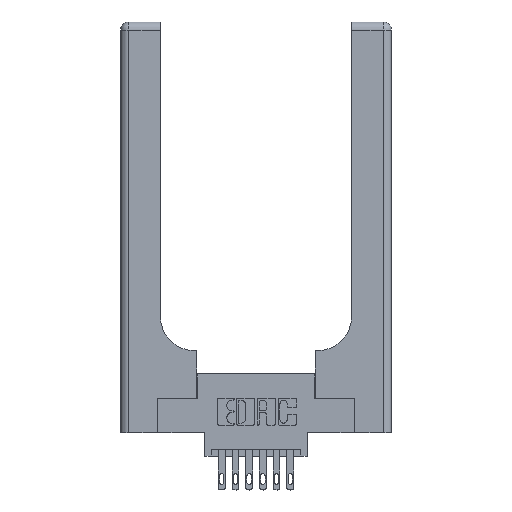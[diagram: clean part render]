
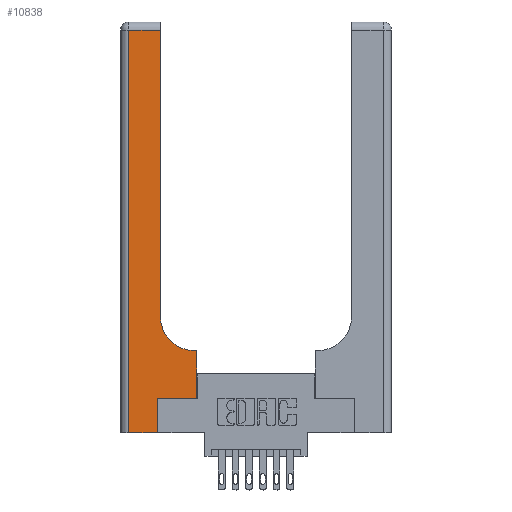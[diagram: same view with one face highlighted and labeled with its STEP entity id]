
A CAD part, top view. The second image highlights one B-rep face of the part: STEP entity #10838.
In plain terms, the highlighted planar face has unit normal (0, 0, 1).
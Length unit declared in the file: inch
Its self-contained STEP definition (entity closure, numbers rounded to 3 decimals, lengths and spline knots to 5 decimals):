
#20 = CARTESIAN_POINT ( 'NONE',  ( 0.2915, 0.6, 0.37 ) ) ;
#123 = PLANE ( 'NONE',  #11842 ) ;
#277 = CARTESIAN_POINT ( 'NONE',  ( 0.06, 0., 0.37 ) ) ;
#364 = EDGE_CURVE ( 'NONE', #12916, #10459, #4195, .T. ) ;
#506 = VECTOR ( 'NONE', #4941, 39.37008 ) ;
#641 = DIRECTION ( 'NONE',  ( 0., 1., 0. ) ) ;
#642 = EDGE_CURVE ( 'NONE', #7606, #8625, #7734, .T. ) ;
#689 = ORIENTED_EDGE ( 'NONE', *, *, #13143, .T. ) ;
#732 = VECTOR ( 'NONE', #7771, 39.37008 ) ;
#889 = DIRECTION ( 'NONE',  ( -1., 0., 0. ) ) ;
#1004 = ORIENTED_EDGE ( 'NONE', *, *, #14574, .T. ) ;
#1113 = VECTOR ( 'NONE', #1966, 39.37008 ) ;
#1472 = CARTESIAN_POINT ( 'NONE',  ( 0.5415, 0.6, 0.37 ) ) ;
#1966 = DIRECTION ( 'NONE',  ( 1., 0., 0. ) ) ;
#2055 = ORIENTED_EDGE ( 'NONE', *, *, #12424, .T. ) ;
#2529 = VECTOR ( 'NONE', #12129, 39.37008 ) ;
#2734 = VERTEX_POINT ( 'NONE', #10168 ) ;
#2869 = ORIENTED_EDGE ( 'NONE', *, *, #642, .T. ) ;
#3172 = EDGE_CURVE ( 'NONE', #13018, #13622, #7859, .T. ) ;
#3387 = CARTESIAN_POINT ( 'NONE',  ( 0.269, 0., 0.37 ) ) ;
#4195 = CIRCLE ( 'NONE', #6456, 0.25 ) ;
#4466 = VECTOR ( 'NONE', #641, 39.37008 ) ;
#4496 = LINE ( 'NONE', #20, #12321 ) ;
#4925 = CARTESIAN_POINT ( 'NONE',  ( 0.5585, 0.25, 0.37 ) ) ;
#4941 = DIRECTION ( 'NONE',  ( 1., 0., 0. ) ) ;
#5006 = LINE ( 'NONE', #11757, #506 ) ;
#5586 = LINE ( 'NONE', #11095, #732 ) ;
#5652 = DIRECTION ( 'NONE',  ( 1., 0., 0. ) ) ;
#6067 = LINE ( 'NONE', #12488, #12828 ) ;
#6456 = AXIS2_PLACEMENT_3D ( 'NONE', #11412, #7791, #5652 ) ;
#6542 = ORIENTED_EDGE ( 'NONE', *, *, #14166, .T. ) ;
#7606 = VERTEX_POINT ( 'NONE', #277 ) ;
#7608 = CARTESIAN_POINT ( 'NONE',  ( 0.06, 3., 0.37 ) ) ;
#7734 = LINE ( 'NONE', #13352, #1113 ) ;
#7771 = DIRECTION ( 'NONE',  ( 0., 1., 0. ) ) ;
#7791 = DIRECTION ( 'NONE',  ( 0., 0., -1. ) ) ;
#7859 = LINE ( 'NONE', #10879, #4466 ) ;
#8048 = DIRECTION ( 'NONE',  ( -1., 0., 0. ) ) ;
#8280 = CARTESIAN_POINT ( 'NONE',  ( 0.06, 2.94, 0.37 ) ) ;
#8443 = CARTESIAN_POINT ( 'NONE',  ( 0.5585, 0.6, 0.37 ) ) ;
#8625 = VERTEX_POINT ( 'NONE', #3387 ) ;
#8640 = EDGE_LOOP ( 'NONE', ( #2055, #689, #12978, #2869, #1004, #6542, #13988, #13769, #12997 ) ) ;
#8999 = CARTESIAN_POINT ( 'NONE',  ( 0., 2.94, 0.37 ) ) ;
#9202 = FACE_OUTER_BOUND ( 'NONE', #8640, .T. ) ;
#9397 = CARTESIAN_POINT ( 'NONE',  ( 0., 3., 0.37 ) ) ;
#9447 = DIRECTION ( 'NONE',  ( 0., 0., -1. ) ) ;
#9547 = EDGE_CURVE ( 'NONE', #12244, #7606, #11401, .T. ) ;
#9946 = VERTEX_POINT ( 'NONE', #13334 ) ;
#10096 = DIRECTION ( 'NONE',  ( 0., 1., 0. ) ) ;
#10168 = CARTESIAN_POINT ( 'NONE',  ( 0.269, 0.25, 0.37 ) ) ;
#10459 = VERTEX_POINT ( 'NONE', #14615 ) ;
#10838 = ADVANCED_FACE ( 'NONE', ( #9202 ), #123, .F. ) ;
#10879 = CARTESIAN_POINT ( 'NONE',  ( 0.5585, 0.25, 0.37 ) ) ;
#11095 = CARTESIAN_POINT ( 'NONE',  ( 0.2915, 3., 0.37 ) ) ;
#11401 = LINE ( 'NONE', #7608, #2529 ) ;
#11412 = CARTESIAN_POINT ( 'NONE',  ( 0.5415, 0.85, 0.37 ) ) ;
#11757 = CARTESIAN_POINT ( 'NONE',  ( 0.269, 0.25, 0.37 ) ) ;
#11842 = AXIS2_PLACEMENT_3D ( 'NONE', #9397, #9447, #12721 ) ;
#12129 = DIRECTION ( 'NONE',  ( 0., -1., 0. ) ) ;
#12244 = VERTEX_POINT ( 'NONE', #8280 ) ;
#12321 = VECTOR ( 'NONE', #8048, 39.37008 ) ;
#12424 = EDGE_CURVE ( 'NONE', #10459, #9946, #5586, .T. ) ;
#12488 = CARTESIAN_POINT ( 'NONE',  ( 0.269, 0., 0.37 ) ) ;
#12721 = DIRECTION ( 'NONE',  ( -1., 0., 0. ) ) ;
#12828 = VECTOR ( 'NONE', #10096, 39.37008 ) ;
#12916 = VERTEX_POINT ( 'NONE', #1472 ) ;
#12978 = ORIENTED_EDGE ( 'NONE', *, *, #9547, .T. ) ;
#12997 = ORIENTED_EDGE ( 'NONE', *, *, #364, .T. ) ;
#13018 = VERTEX_POINT ( 'NONE', #4925 ) ;
#13143 = EDGE_CURVE ( 'NONE', #9946, #12244, #13556, .T. ) ;
#13212 = VECTOR ( 'NONE', #889, 39.37008 ) ;
#13328 = EDGE_CURVE ( 'NONE', #13622, #12916, #4496, .T. ) ;
#13334 = CARTESIAN_POINT ( 'NONE',  ( 0.2915, 2.94, 0.37 ) ) ;
#13352 = CARTESIAN_POINT ( 'NONE',  ( 0., 0., 0.37 ) ) ;
#13556 = LINE ( 'NONE', #8999, #13212 ) ;
#13622 = VERTEX_POINT ( 'NONE', #8443 ) ;
#13769 = ORIENTED_EDGE ( 'NONE', *, *, #13328, .T. ) ;
#13988 = ORIENTED_EDGE ( 'NONE', *, *, #3172, .T. ) ;
#14166 = EDGE_CURVE ( 'NONE', #2734, #13018, #5006, .T. ) ;
#14574 = EDGE_CURVE ( 'NONE', #8625, #2734, #6067, .T. ) ;
#14615 = CARTESIAN_POINT ( 'NONE',  ( 0.2915, 0.85, 0.37 ) ) ;
